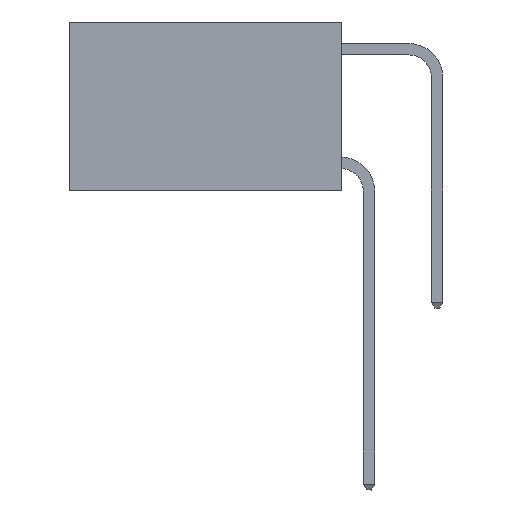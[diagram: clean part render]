
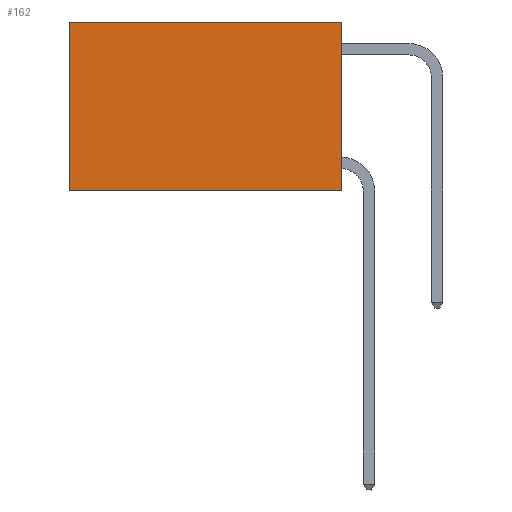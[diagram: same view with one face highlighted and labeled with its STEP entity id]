
A CAD part, left-side view. The second image highlights one B-rep face of the part: STEP entity #162.
In plain terms, the highlighted planar face has unit normal (-1, 0, 0).
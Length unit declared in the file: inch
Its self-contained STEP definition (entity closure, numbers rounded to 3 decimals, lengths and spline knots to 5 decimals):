
#162 = ADVANCED_FACE ( 'NONE', ( #14767 ), #5722, .F. ) ;
#989 = VECTOR ( 'NONE', #15925, 39.37008 ) ;
#1465 = LINE ( 'NONE', #12877, #989 ) ;
#2329 = DIRECTION ( 'NONE',  ( 0., 1., 0. ) ) ;
#2599 = CARTESIAN_POINT ( 'NONE',  ( 0.2625, 0., 0. ) ) ;
#3247 = EDGE_CURVE ( 'NONE', #7240, #6887, #11106, .T. ) ;
#3873 = CARTESIAN_POINT ( 'NONE',  ( 0.2625, 0., 0. ) ) ;
#5602 = VERTEX_POINT ( 'NONE', #15743 ) ;
#5722 = PLANE ( 'NONE',  #19431 ) ;
#6845 = CARTESIAN_POINT ( 'NONE',  ( 0.2625, 0., -0.37 ) ) ;
#6887 = VERTEX_POINT ( 'NONE', #10637 ) ;
#7240 = VERTEX_POINT ( 'NONE', #6845 ) ;
#7561 = ORIENTED_EDGE ( 'NONE', *, *, #15053, .T. ) ;
#7705 = CARTESIAN_POINT ( 'NONE',  ( 0.2625, 0., 0. ) ) ;
#8683 = CARTESIAN_POINT ( 'NONE',  ( 0.2625, 0., -0.37 ) ) ;
#9442 = EDGE_LOOP ( 'NONE', ( #7561, #10316, #12796, #18755 ) ) ;
#10016 = DIRECTION ( 'NONE',  ( 0., 0., -1. ) ) ;
#10316 = ORIENTED_EDGE ( 'NONE', *, *, #3247, .F. ) ;
#10594 = VECTOR ( 'NONE', #17682, 39.37008 ) ;
#10637 = CARTESIAN_POINT ( 'NONE',  ( 0.2625, 0.6, -0.37 ) ) ;
#11106 = LINE ( 'NONE', #8683, #18182 ) ;
#12498 = EDGE_CURVE ( 'NONE', #5602, #7240, #14581, .T. ) ;
#12770 = CARTESIAN_POINT ( 'NONE',  ( 0.2625, 0.6, 0. ) ) ;
#12796 = ORIENTED_EDGE ( 'NONE', *, *, #12498, .F. ) ;
#12877 = CARTESIAN_POINT ( 'NONE',  ( 0.2625, 0.6, 0. ) ) ;
#14581 = LINE ( 'NONE', #2599, #10594 ) ;
#14767 = FACE_OUTER_BOUND ( 'NONE', #9442, .T. ) ;
#15053 = EDGE_CURVE ( 'NONE', #19123, #6887, #1465, .T. ) ;
#15743 = CARTESIAN_POINT ( 'NONE',  ( 0.2625, 0., 0. ) ) ;
#15751 = EDGE_CURVE ( 'NONE', #5602, #19123, #17798, .T. ) ;
#15925 = DIRECTION ( 'NONE',  ( 0., 0., -1. ) ) ;
#17325 = VECTOR ( 'NONE', #2329, 39.37008 ) ;
#17682 = DIRECTION ( 'NONE',  ( 0., 0., -1. ) ) ;
#17798 = LINE ( 'NONE', #3873, #17325 ) ;
#18182 = VECTOR ( 'NONE', #19295, 39.37008 ) ;
#18755 = ORIENTED_EDGE ( 'NONE', *, *, #15751, .T. ) ;
#19123 = VERTEX_POINT ( 'NONE', #12770 ) ;
#19295 = DIRECTION ( 'NONE',  ( 0., 1., 0. ) ) ;
#19431 = AXIS2_PLACEMENT_3D ( 'NONE', #7705, #19607, #10016 ) ;
#19607 = DIRECTION ( 'NONE',  ( 1., 0., 0. ) ) ;
